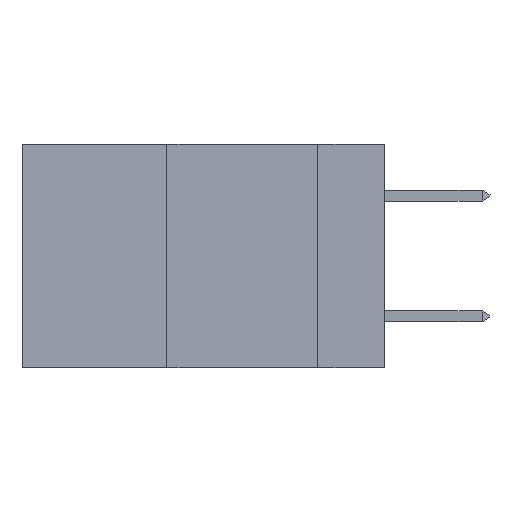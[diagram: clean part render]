
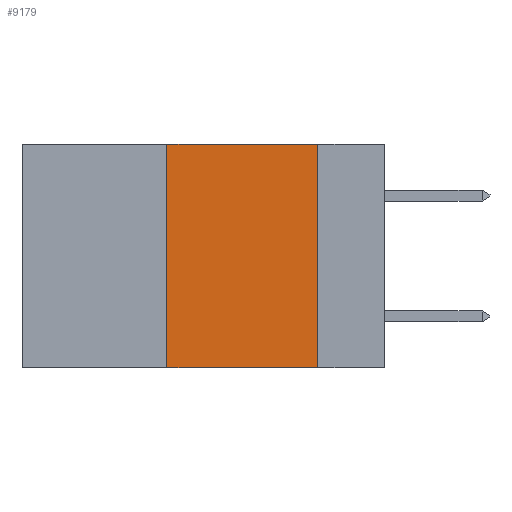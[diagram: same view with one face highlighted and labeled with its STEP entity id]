
A CAD part, left-side view. The second image highlights one B-rep face of the part: STEP entity #9179.
In plain terms, the highlighted planar face has unit normal (-1, 0, 0).
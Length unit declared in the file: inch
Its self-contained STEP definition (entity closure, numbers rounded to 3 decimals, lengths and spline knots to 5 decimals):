
#608 = DIRECTION ( 'NONE',  ( 0., 0., 1. ) ) ;
#1379 = ORIENTED_EDGE ( 'NONE', *, *, #9482, .T. ) ;
#2132 = AXIS2_PLACEMENT_3D ( 'NONE', #9634, #14579, #3230 ) ;
#2580 = VECTOR ( 'NONE', #3008, 39.37008 ) ;
#2852 = VERTEX_POINT ( 'NONE', #12265 ) ;
#2875 = ORIENTED_EDGE ( 'NONE', *, *, #13095, .F. ) ;
#3008 = DIRECTION ( 'NONE',  ( 0., 0., -1. ) ) ;
#3013 = VECTOR ( 'NONE', #608, 39.37008 ) ;
#3230 = DIRECTION ( 'NONE',  ( 0., 0., -1. ) ) ;
#3270 = VECTOR ( 'NONE', #9695, 39.37008 ) ;
#4387 = EDGE_LOOP ( 'NONE', ( #16027, #12462, #2875, #1379 ) ) ;
#4509 = VERTEX_POINT ( 'NONE', #5208 ) ;
#5208 = CARTESIAN_POINT ( 'NONE',  ( 0., 0.11, 0. ) ) ;
#6002 = FACE_OUTER_BOUND ( 'NONE', #4387, .T. ) ;
#6233 = CARTESIAN_POINT ( 'NONE',  ( 0., 0.36, -0.37 ) ) ;
#6359 = VERTEX_POINT ( 'NONE', #9122 ) ;
#6648 = LINE ( 'NONE', #14684, #3270 ) ;
#6917 = CARTESIAN_POINT ( 'NONE',  ( 0., 0.36, 0. ) ) ;
#7215 = CARTESIAN_POINT ( 'NONE',  ( 0., 0.6, -0.37 ) ) ;
#8112 = EDGE_CURVE ( 'NONE', #2852, #4509, #6648, .T. ) ;
#8501 = DIRECTION ( 'NONE',  ( 0., -1., 0. ) ) ;
#8762 = LINE ( 'NONE', #6917, #3013 ) ;
#9122 = CARTESIAN_POINT ( 'NONE',  ( 0., 0.11, -0.37 ) ) ;
#9179 = ADVANCED_FACE ( 'NONE', ( #6002 ), #13461, .F. ) ;
#9482 = EDGE_CURVE ( 'NONE', #16218, #6359, #13866, .T. ) ;
#9634 = CARTESIAN_POINT ( 'NONE',  ( 0., 0.6, 0. ) ) ;
#9695 = DIRECTION ( 'NONE',  ( 0., -1., 0. ) ) ;
#10075 = LINE ( 'NONE', #13195, #2580 ) ;
#10542 = VECTOR ( 'NONE', #8501, 39.37008 ) ;
#10979 = EDGE_CURVE ( 'NONE', #4509, #6359, #10075, .T. ) ;
#12265 = CARTESIAN_POINT ( 'NONE',  ( 0., 0.36, 0. ) ) ;
#12462 = ORIENTED_EDGE ( 'NONE', *, *, #8112, .F. ) ;
#13095 = EDGE_CURVE ( 'NONE', #16218, #2852, #8762, .T. ) ;
#13195 = CARTESIAN_POINT ( 'NONE',  ( 0., 0.11, 0. ) ) ;
#13461 = PLANE ( 'NONE',  #2132 ) ;
#13866 = LINE ( 'NONE', #7215, #10542 ) ;
#14579 = DIRECTION ( 'NONE',  ( 1., 0., 0. ) ) ;
#14684 = CARTESIAN_POINT ( 'NONE',  ( 0., 0.6, 0. ) ) ;
#16027 = ORIENTED_EDGE ( 'NONE', *, *, #10979, .F. ) ;
#16218 = VERTEX_POINT ( 'NONE', #6233 ) ;
